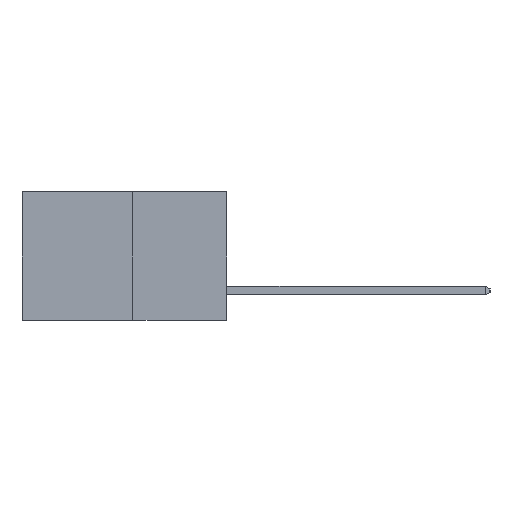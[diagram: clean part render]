
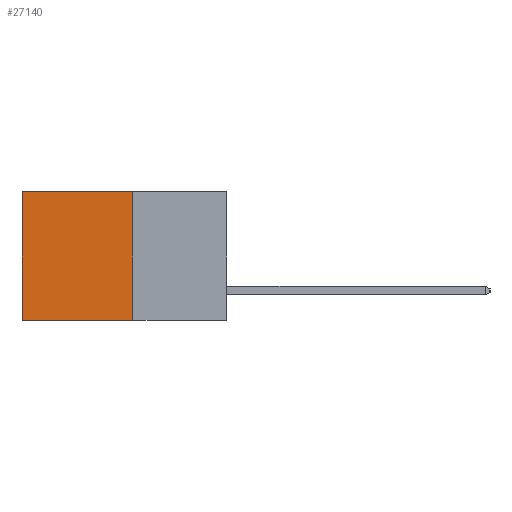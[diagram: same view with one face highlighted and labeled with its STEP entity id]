
A CAD part, left-side view. The second image highlights one B-rep face of the part: STEP entity #27140.
In plain terms, the highlighted planar face has unit normal (-1, 0, 0).
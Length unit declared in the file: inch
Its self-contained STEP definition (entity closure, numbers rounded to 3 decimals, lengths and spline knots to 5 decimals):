
#382 = VECTOR ( 'NONE', #31955, 39.37008 ) ;
#654 = CARTESIAN_POINT ( 'NONE',  ( 0.277, 0.27, 0. ) ) ;
#1288 = VERTEX_POINT ( 'NONE', #25889 ) ;
#1948 = VERTEX_POINT ( 'NONE', #654 ) ;
#2058 = PLANE ( 'NONE',  #7224 ) ;
#3162 = CARTESIAN_POINT ( 'NONE',  ( 0.277, 0.59, 0. ) ) ;
#5652 = ORIENTED_EDGE ( 'NONE', *, *, #30359, .T. ) ;
#6967 = ORIENTED_EDGE ( 'NONE', *, *, #24427, .F. ) ;
#7224 = AXIS2_PLACEMENT_3D ( 'NONE', #25326, #9957, #27889 ) ;
#7724 = DIRECTION ( 'NONE',  ( 0., 0., -1. ) ) ;
#7725 = DIRECTION ( 'NONE',  ( 0., 1., 0. ) ) ;
#7940 = EDGE_CURVE ( 'NONE', #15685, #1288, #11450, .T. ) ;
#9296 = DIRECTION ( 'NONE',  ( 0., 0., -1. ) ) ;
#9708 = CARTESIAN_POINT ( 'NONE',  ( 0.277, 0.59, -0.37 ) ) ;
#9957 = DIRECTION ( 'NONE',  ( 1., 0., 0. ) ) ;
#11450 = LINE ( 'NONE', #9708, #24301 ) ;
#11526 = CARTESIAN_POINT ( 'NONE',  ( 0.277, 0.27, -0.37 ) ) ;
#14028 = LINE ( 'NONE', #11526, #382 ) ;
#14375 = FACE_OUTER_BOUND ( 'NONE', #20005, .T. ) ;
#15685 = VERTEX_POINT ( 'NONE', #3162 ) ;
#17251 = ORIENTED_EDGE ( 'NONE', *, *, #7940, .T. ) ;
#17950 = CARTESIAN_POINT ( 'NONE',  ( 0.277, 0.27, -0.37 ) ) ;
#20005 = EDGE_LOOP ( 'NONE', ( #17251, #6967, #32414, #5652 ) ) ;
#20508 = CARTESIAN_POINT ( 'NONE',  ( 0.277, 0.27, 0. ) ) ;
#23405 = VECTOR ( 'NONE', #7725, 39.37008 ) ;
#24301 = VECTOR ( 'NONE', #9296, 39.37008 ) ;
#24427 = EDGE_CURVE ( 'NONE', #29783, #1288, #14028, .T. ) ;
#25318 = LINE ( 'NONE', #17950, #31264 ) ;
#25326 = CARTESIAN_POINT ( 'NONE',  ( 0.277, 0.27, -0.37 ) ) ;
#25889 = CARTESIAN_POINT ( 'NONE',  ( 0.277, 0.59, -0.37 ) ) ;
#25939 = CARTESIAN_POINT ( 'NONE',  ( 0.277, 0.27, -0.37 ) ) ;
#26087 = EDGE_CURVE ( 'NONE', #1948, #29783, #25318, .T. ) ;
#27140 = ADVANCED_FACE ( 'NONE', ( #14375 ), #2058, .F. ) ;
#27889 = DIRECTION ( 'NONE',  ( 0., 0., -1. ) ) ;
#29783 = VERTEX_POINT ( 'NONE', #25939 ) ;
#30174 = LINE ( 'NONE', #20508, #23405 ) ;
#30359 = EDGE_CURVE ( 'NONE', #1948, #15685, #30174, .T. ) ;
#31264 = VECTOR ( 'NONE', #7724, 39.37008 ) ;
#31955 = DIRECTION ( 'NONE',  ( 0., 1., 0. ) ) ;
#32414 = ORIENTED_EDGE ( 'NONE', *, *, #26087, .F. ) ;
